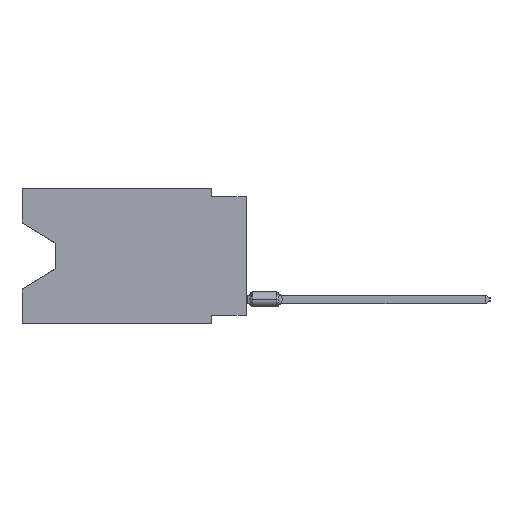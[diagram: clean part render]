
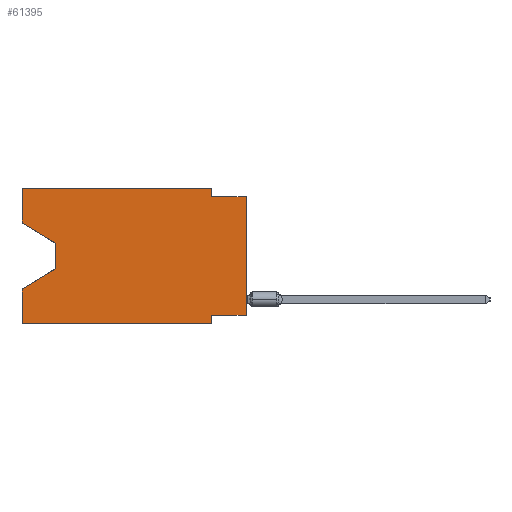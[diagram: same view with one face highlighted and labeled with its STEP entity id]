
A CAD part, left-side view. The second image highlights one B-rep face of the part: STEP entity #61395.
In plain terms, the highlighted planar face has unit normal (-1, 0, 0).
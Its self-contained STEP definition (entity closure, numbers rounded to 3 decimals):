
#2068 = VERTEX_POINT ( 'NONE', #74290 ) ;
#3107 = ORIENTED_EDGE ( 'NONE', *, *, #70333, .F. ) ;
#4143 = DIRECTION ( 'NONE',  ( 0., 0.855, -0.519 ) ) ;
#4555 = CARTESIAN_POINT ( 'NONE',  ( 0., 13.97, -5.893 ) ) ;
#4728 = EDGE_CURVE ( 'NONE', #2068, #68510, #37087, .T. ) ;
#4795 = DIRECTION ( 'NONE',  ( 0., -1., 0. ) ) ;
#4968 = CARTESIAN_POINT ( 'NONE',  ( 0., 0., 0. ) ) ;
#5384 = EDGE_CURVE ( 'NONE', #59886, #49013, #42747, .T. ) ;
#6213 = CARTESIAN_POINT ( 'NONE',  ( 0., 2.54, -9.271 ) ) ;
#6410 = VECTOR ( 'NONE', #36385, 1000. ) ;
#6790 = CARTESIAN_POINT ( 'NONE',  ( 0., 16.383, 0. ) ) ;
#8347 = VERTEX_POINT ( 'NONE', #67796 ) ;
#8540 = CARTESIAN_POINT ( 'NONE',  ( 0., 16.383, 0. ) ) ;
#10105 = DIRECTION ( 'NONE',  ( 0., -0.855, -0.519 ) ) ;
#12142 = DIRECTION ( 'NONE',  ( 0., 0., -1. ) ) ;
#12410 = ORIENTED_EDGE ( 'NONE', *, *, #4728, .F. ) ;
#12544 = ORIENTED_EDGE ( 'NONE', *, *, #40459, .F. ) ;
#12666 = CARTESIAN_POINT ( 'NONE',  ( 0., 2.54, 0. ) ) ;
#12963 = CARTESIAN_POINT ( 'NONE',  ( 0., 13.97, -4.013 ) ) ;
#13241 = CARTESIAN_POINT ( 'NONE',  ( 0., 2.54, -0.635 ) ) ;
#15309 = PLANE ( 'NONE',  #46972 ) ;
#16415 = CARTESIAN_POINT ( 'NONE',  ( 0., 16.383, -7.36 ) ) ;
#17612 = ORIENTED_EDGE ( 'NONE', *, *, #38740, .F. ) ;
#18496 = DIRECTION ( 'NONE',  ( 0., 0., -1. ) ) ;
#21048 = LINE ( 'NONE', #27833, #65852 ) ;
#21433 = VECTOR ( 'NONE', #70180, 1000. ) ;
#21454 = DIRECTION ( 'NONE',  ( 0., 0., 1. ) ) ;
#24604 = VECTOR ( 'NONE', #18496, 1000. ) ;
#25099 = DIRECTION ( 'NONE',  ( 0., -1., 0. ) ) ;
#26352 = VERTEX_POINT ( 'NONE', #6213 ) ;
#27833 = CARTESIAN_POINT ( 'NONE',  ( 0., 16.383, 0. ) ) ;
#28673 = CARTESIAN_POINT ( 'NONE',  ( 0., 0., -9.271 ) ) ;
#29540 = VERTEX_POINT ( 'NONE', #46339 ) ;
#31157 = VERTEX_POINT ( 'NONE', #67803 ) ;
#31946 = CARTESIAN_POINT ( 'NONE',  ( 0., 0., -9.271 ) ) ;
#32208 = DIRECTION ( 'NONE',  ( 0., 0., -1. ) ) ;
#32690 = DIRECTION ( 'NONE',  ( 0., 0., 1. ) ) ;
#33349 = ORIENTED_EDGE ( 'NONE', *, *, #76512, .T. ) ;
#33649 = EDGE_CURVE ( 'NONE', #29540, #44288, #41543, .T. ) ;
#35131 = VERTEX_POINT ( 'NONE', #74998 ) ;
#35262 = VECTOR ( 'NONE', #25099, 1000. ) ;
#36385 = DIRECTION ( 'NONE',  ( 0., -1., 0. ) ) ;
#36844 = ORIENTED_EDGE ( 'NONE', *, *, #33649, .T. ) ;
#37087 = LINE ( 'NONE', #62995, #74166 ) ;
#37249 = LINE ( 'NONE', #4968, #67049 ) ;
#38740 = EDGE_CURVE ( 'NONE', #68510, #59886, #44963, .T. ) ;
#40459 = EDGE_CURVE ( 'NONE', #26352, #31157, #70346, .T. ) ;
#41543 = LINE ( 'NONE', #68278, #64974 ) ;
#42747 = LINE ( 'NONE', #55937, #6410 ) ;
#44288 = VERTEX_POINT ( 'NONE', #82890 ) ;
#44963 = LINE ( 'NONE', #12666, #70134 ) ;
#46339 = CARTESIAN_POINT ( 'NONE',  ( 0., 16.383, -2.546 ) ) ;
#46972 = AXIS2_PLACEMENT_3D ( 'NONE', #8540, #67134, #48035 ) ;
#48035 = DIRECTION ( 'NONE',  ( 0., 0., -1. ) ) ;
#48411 = CARTESIAN_POINT ( 'NONE',  ( 0., 2.54, -9.906 ) ) ;
#49013 = VERTEX_POINT ( 'NONE', #73223 ) ;
#49650 = EDGE_CURVE ( 'NONE', #35131, #31157, #64180, .T. ) ;
#50348 = VERTEX_POINT ( 'NONE', #16415 ) ;
#50680 = LINE ( 'NONE', #6790, #58267 ) ;
#51296 = DIRECTION ( 'NONE',  ( 0., 0., 1. ) ) ;
#55937 = CARTESIAN_POINT ( 'NONE',  ( 0., 0., -0.635 ) ) ;
#56567 = CARTESIAN_POINT ( 'NONE',  ( 0., 16.383, -9.906 ) ) ;
#56943 = ORIENTED_EDGE ( 'NONE', *, *, #78563, .F. ) ;
#57614 = EDGE_CURVE ( 'NONE', #57903, #49013, #37249, .T. ) ;
#57744 = CARTESIAN_POINT ( 'NONE',  ( 0., 2.54, 0. ) ) ;
#57903 = VERTEX_POINT ( 'NONE', #28673 ) ;
#58267 = VECTOR ( 'NONE', #32690, 1000. ) ;
#59886 = VERTEX_POINT ( 'NONE', #13241 ) ;
#61395 = ADVANCED_FACE ( 'NONE', ( #66723 ), #15309, .F. ) ;
#62995 = CARTESIAN_POINT ( 'NONE',  ( 0., 16.383, 0. ) ) ;
#63658 = VECTOR ( 'NONE', #4143, 1000. ) ;
#64180 = LINE ( 'NONE', #56567, #35262 ) ;
#64974 = VECTOR ( 'NONE', #10105, 1000. ) ;
#65852 = VECTOR ( 'NONE', #21454, 1000. ) ;
#66723 = FACE_OUTER_BOUND ( 'NONE', #70194, .T. ) ;
#66792 = VECTOR ( 'NONE', #12142, 1000. ) ;
#67049 = VECTOR ( 'NONE', #51296, 1000. ) ;
#67134 = DIRECTION ( 'NONE',  ( 1., 0., 0. ) ) ;
#67796 = CARTESIAN_POINT ( 'NONE',  ( 0., 13.97, -5.893 ) ) ;
#67803 = CARTESIAN_POINT ( 'NONE',  ( 0., 2.54, -9.906 ) ) ;
#68278 = CARTESIAN_POINT ( 'NONE',  ( 0., 16.383, -2.546 ) ) ;
#68510 = VERTEX_POINT ( 'NONE', #57744 ) ;
#69758 = LINE ( 'NONE', #31946, #21433 ) ;
#70134 = VECTOR ( 'NONE', #32208, 1000. ) ;
#70180 = DIRECTION ( 'NONE',  ( 0., 1., 0. ) ) ;
#70194 = EDGE_LOOP ( 'NONE', ( #36844, #80295, #33349, #3107, #81262, #12544, #76452, #70521, #75719, #17612, #12410, #56943 ) ) ;
#70333 = EDGE_CURVE ( 'NONE', #35131, #50348, #21048, .T. ) ;
#70346 = LINE ( 'NONE', #48411, #66792 ) ;
#70521 = ORIENTED_EDGE ( 'NONE', *, *, #57614, .T. ) ;
#73223 = CARTESIAN_POINT ( 'NONE',  ( 0., 0., -0.635 ) ) ;
#74166 = VECTOR ( 'NONE', #4795, 1000. ) ;
#74290 = CARTESIAN_POINT ( 'NONE',  ( 0., 16.383, 0. ) ) ;
#74998 = CARTESIAN_POINT ( 'NONE',  ( 0., 16.383, -9.906 ) ) ;
#75415 = EDGE_CURVE ( 'NONE', #57903, #26352, #69758, .T. ) ;
#75719 = ORIENTED_EDGE ( 'NONE', *, *, #5384, .F. ) ;
#76452 = ORIENTED_EDGE ( 'NONE', *, *, #75415, .F. ) ;
#76512 = EDGE_CURVE ( 'NONE', #8347, #50348, #81877, .T. ) ;
#78563 = EDGE_CURVE ( 'NONE', #29540, #2068, #50680, .T. ) ;
#80295 = ORIENTED_EDGE ( 'NONE', *, *, #81840, .T. ) ;
#81262 = ORIENTED_EDGE ( 'NONE', *, *, #49650, .T. ) ;
#81840 = EDGE_CURVE ( 'NONE', #44288, #8347, #83070, .T. ) ;
#81877 = LINE ( 'NONE', #4555, #63658 ) ;
#82890 = CARTESIAN_POINT ( 'NONE',  ( 0., 13.97, -4.013 ) ) ;
#83070 = LINE ( 'NONE', #12963, #24604 ) ;
